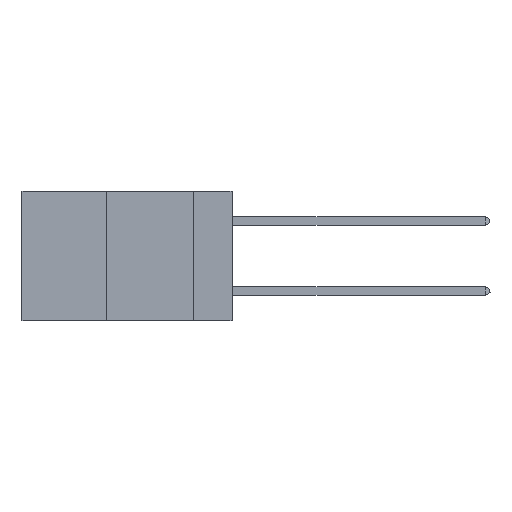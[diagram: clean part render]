
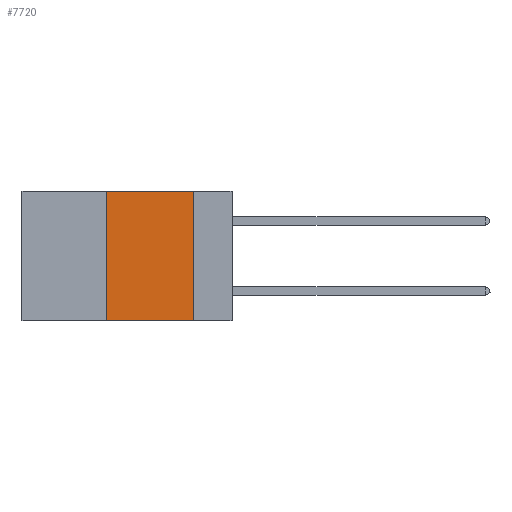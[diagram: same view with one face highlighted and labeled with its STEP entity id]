
A CAD part, left-side view. The second image highlights one B-rep face of the part: STEP entity #7720.
In plain terms, the highlighted planar face has unit normal (-1, 0, 0).
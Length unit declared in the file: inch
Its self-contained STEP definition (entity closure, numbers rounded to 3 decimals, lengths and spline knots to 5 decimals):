
#59 = DIRECTION ( 'NONE',  ( 0., 0., -1. ) ) ;
#335 = ORIENTED_EDGE ( 'NONE', *, *, #6260, .F. ) ;
#652 = ORIENTED_EDGE ( 'NONE', *, *, #10361, .F. ) ;
#832 = DIRECTION ( 'NONE',  ( 0., 0., -1. ) ) ;
#1627 = DIRECTION ( 'NONE',  ( 0., -1., 0. ) ) ;
#2297 = ORIENTED_EDGE ( 'NONE', *, *, #12213, .F. ) ;
#2716 = CARTESIAN_POINT ( 'NONE',  ( 0., 0.36, -0.37 ) ) ;
#3163 = EDGE_LOOP ( 'NONE', ( #335, #652, #2297, #3501 ) ) ;
#3501 = ORIENTED_EDGE ( 'NONE', *, *, #4753, .T. ) ;
#3952 = LINE ( 'NONE', #6420, #6126 ) ;
#4318 = VECTOR ( 'NONE', #9474, 39.37008 ) ;
#4666 = CARTESIAN_POINT ( 'NONE',  ( 0., 0.11, 0. ) ) ;
#4753 = EDGE_CURVE ( 'NONE', #6835, #10434, #11682, .T. ) ;
#5025 = FACE_OUTER_BOUND ( 'NONE', #3163, .T. ) ;
#5061 = PLANE ( 'NONE',  #9695 ) ;
#5994 = DIRECTION ( 'NONE',  ( 1., 0., 0. ) ) ;
#6077 = VECTOR ( 'NONE', #7874, 39.37008 ) ;
#6126 = VECTOR ( 'NONE', #1627, 39.37008 ) ;
#6260 = EDGE_CURVE ( 'NONE', #9586, #10434, #8694, .T. ) ;
#6420 = CARTESIAN_POINT ( 'NONE',  ( 0., 0.6, 0. ) ) ;
#6835 = VERTEX_POINT ( 'NONE', #2716 ) ;
#7720 = ADVANCED_FACE ( 'NONE', ( #5025 ), #5061, .F. ) ;
#7874 = DIRECTION ( 'NONE',  ( 0., 0., 1. ) ) ;
#8285 = CARTESIAN_POINT ( 'NONE',  ( 0., 0.11, 0. ) ) ;
#8414 = VECTOR ( 'NONE', #832, 39.37008 ) ;
#8612 = LINE ( 'NONE', #8812, #6077 ) ;
#8694 = LINE ( 'NONE', #4666, #8414 ) ;
#8812 = CARTESIAN_POINT ( 'NONE',  ( 0., 0.36, 0. ) ) ;
#8822 = VERTEX_POINT ( 'NONE', #9205 ) ;
#8825 = CARTESIAN_POINT ( 'NONE',  ( 0., 0.6, 0. ) ) ;
#9205 = CARTESIAN_POINT ( 'NONE',  ( 0., 0.36, 0. ) ) ;
#9474 = DIRECTION ( 'NONE',  ( 0., -1., 0. ) ) ;
#9586 = VERTEX_POINT ( 'NONE', #8285 ) ;
#9639 = CARTESIAN_POINT ( 'NONE',  ( 0., 0.6, -0.37 ) ) ;
#9695 = AXIS2_PLACEMENT_3D ( 'NONE', #8825, #5994, #59 ) ;
#10211 = CARTESIAN_POINT ( 'NONE',  ( 0., 0.11, -0.37 ) ) ;
#10361 = EDGE_CURVE ( 'NONE', #8822, #9586, #3952, .T. ) ;
#10434 = VERTEX_POINT ( 'NONE', #10211 ) ;
#11682 = LINE ( 'NONE', #9639, #4318 ) ;
#12213 = EDGE_CURVE ( 'NONE', #6835, #8822, #8612, .T. ) ;
